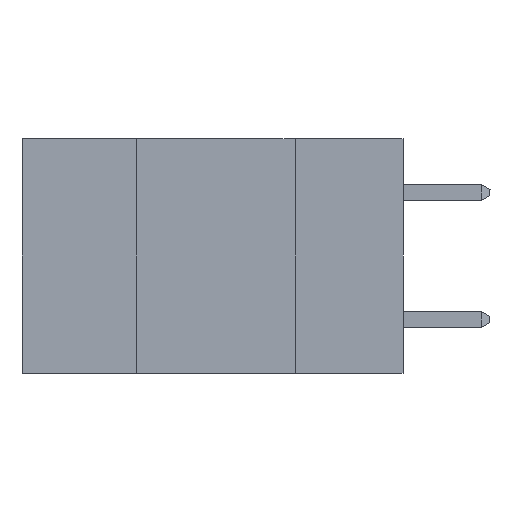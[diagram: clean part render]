
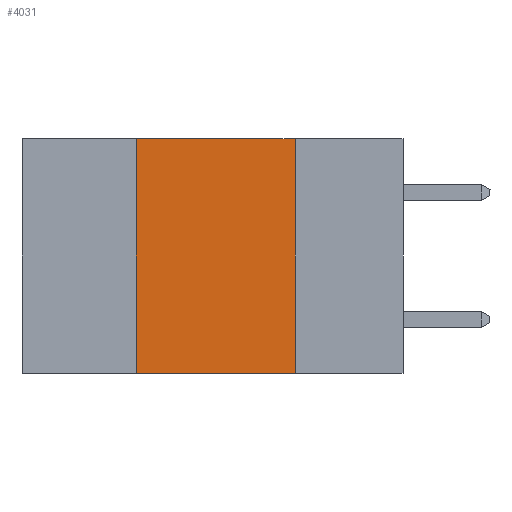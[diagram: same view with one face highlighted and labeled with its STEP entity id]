
A CAD part, left-side view. The second image highlights one B-rep face of the part: STEP entity #4031.
In plain terms, the highlighted planar face has unit normal (-1, 0, 0).
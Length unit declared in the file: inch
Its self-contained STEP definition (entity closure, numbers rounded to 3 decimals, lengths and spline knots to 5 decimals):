
#399 = VERTEX_POINT ( 'NONE', #15705 ) ;
#1265 = ORIENTED_EDGE ( 'NONE', *, *, #8697, .F. ) ;
#1663 = VECTOR ( 'NONE', #9136, 39.37008 ) ;
#3884 = VECTOR ( 'NONE', #4662, 39.37008 ) ;
#4031 = ADVANCED_FACE ( 'NONE', ( #18970 ), #4370, .F. ) ;
#4307 = DIRECTION ( 'NONE',  ( 0., -1., 0. ) ) ;
#4370 = PLANE ( 'NONE',  #6269 ) ;
#4470 = LINE ( 'NONE', #6272, #3884 ) ;
#4662 = DIRECTION ( 'NONE',  ( 0., -1., 0. ) ) ;
#6269 = AXIS2_PLACEMENT_3D ( 'NONE', #16934, #18705, #8016 ) ;
#6272 = CARTESIAN_POINT ( 'NONE',  ( 0., 0.6, 0. ) ) ;
#6456 = VECTOR ( 'NONE', #19419, 39.37008 ) ;
#6479 = CARTESIAN_POINT ( 'NONE',  ( 0., 0.42, -0.37 ) ) ;
#6881 = EDGE_CURVE ( 'NONE', #8523, #19169, #11316, .T. ) ;
#6948 = CARTESIAN_POINT ( 'NONE',  ( 0., 0.17, 0. ) ) ;
#8016 = DIRECTION ( 'NONE',  ( 0., 0., -1. ) ) ;
#8278 = VERTEX_POINT ( 'NONE', #9654 ) ;
#8523 = VERTEX_POINT ( 'NONE', #6479 ) ;
#8697 = EDGE_CURVE ( 'NONE', #399, #8278, #11226, .T. ) ;
#9136 = DIRECTION ( 'NONE',  ( 0., 0., 1. ) ) ;
#9654 = CARTESIAN_POINT ( 'NONE',  ( 0., 0.17, -0.37 ) ) ;
#9904 = EDGE_CURVE ( 'NONE', #19169, #399, #4470, .T. ) ;
#10160 = ORIENTED_EDGE ( 'NONE', *, *, #21630, .T. ) ;
#11226 = LINE ( 'NONE', #6948, #6456 ) ;
#11316 = LINE ( 'NONE', #12652, #1663 ) ;
#12652 = CARTESIAN_POINT ( 'NONE',  ( 0., 0.42, 0. ) ) ;
#15705 = CARTESIAN_POINT ( 'NONE',  ( 0., 0.17, 0. ) ) ;
#16934 = CARTESIAN_POINT ( 'NONE',  ( 0., 0.6, 0. ) ) ;
#18282 = LINE ( 'NONE', #20337, #22398 ) ;
#18705 = DIRECTION ( 'NONE',  ( 1., 0., 0. ) ) ;
#18970 = FACE_OUTER_BOUND ( 'NONE', #20601, .T. ) ;
#19169 = VERTEX_POINT ( 'NONE', #21573 ) ;
#19294 = ORIENTED_EDGE ( 'NONE', *, *, #9904, .F. ) ;
#19419 = DIRECTION ( 'NONE',  ( 0., 0., -1. ) ) ;
#20337 = CARTESIAN_POINT ( 'NONE',  ( 0., 0.6, -0.37 ) ) ;
#20601 = EDGE_LOOP ( 'NONE', ( #1265, #19294, #22331, #10160 ) ) ;
#21573 = CARTESIAN_POINT ( 'NONE',  ( 0., 0.42, 0. ) ) ;
#21630 = EDGE_CURVE ( 'NONE', #8523, #8278, #18282, .T. ) ;
#22331 = ORIENTED_EDGE ( 'NONE', *, *, #6881, .F. ) ;
#22398 = VECTOR ( 'NONE', #4307, 39.37008 ) ;
